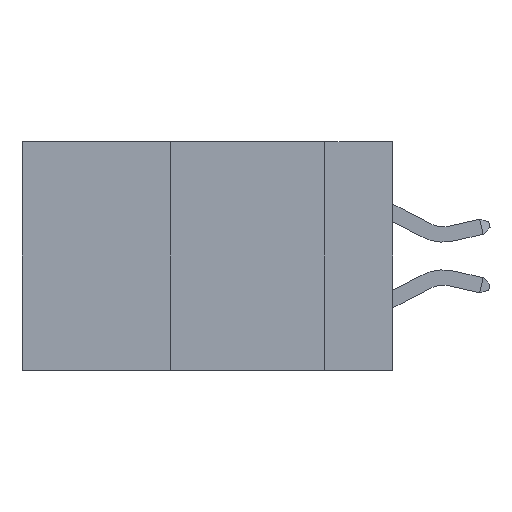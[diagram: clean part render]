
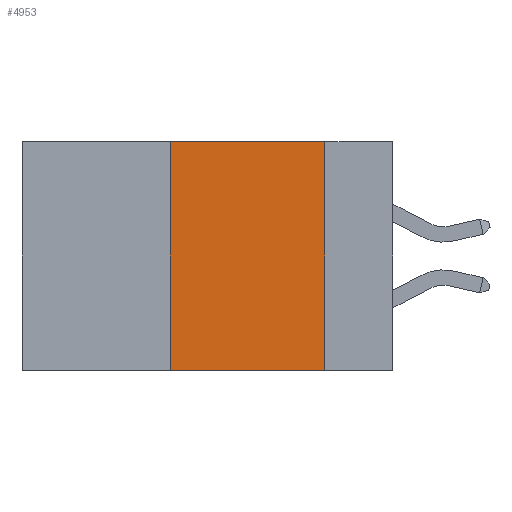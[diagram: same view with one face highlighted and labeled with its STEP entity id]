
A CAD part, left-side view. The second image highlights one B-rep face of the part: STEP entity #4953.
In plain terms, the highlighted planar face has unit normal (-1, 0, 0).
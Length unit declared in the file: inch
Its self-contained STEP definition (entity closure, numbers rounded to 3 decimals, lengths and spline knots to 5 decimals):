
#217 = DIRECTION ( 'NONE',  ( 1., 0., 0. ) ) ;
#533 = CARTESIAN_POINT ( 'NONE',  ( 0., 0.36, -0.37 ) ) ;
#1213 = VERTEX_POINT ( 'NONE', #14336 ) ;
#1267 = DIRECTION ( 'NONE',  ( 0., 0., -1. ) ) ;
#1674 = VECTOR ( 'NONE', #2005, 39.37008 ) ;
#1988 = ORIENTED_EDGE ( 'NONE', *, *, #5839, .F. ) ;
#2005 = DIRECTION ( 'NONE',  ( 0., 0., 1. ) ) ;
#2883 = CARTESIAN_POINT ( 'NONE',  ( 0., 0.36, 0. ) ) ;
#3218 = LINE ( 'NONE', #13666, #1674 ) ;
#3260 = AXIS2_PLACEMENT_3D ( 'NONE', #10325, #217, #1267 ) ;
#3379 = DIRECTION ( 'NONE',  ( 0., -1., 0. ) ) ;
#4046 = EDGE_CURVE ( 'NONE', #10548, #1213, #14669, .T. ) ;
#4181 = EDGE_CURVE ( 'NONE', #4638, #10483, #10303, .T. ) ;
#4638 = VERTEX_POINT ( 'NONE', #533 ) ;
#4953 = ADVANCED_FACE ( 'NONE', ( #10400 ), #5957, .F. ) ;
#5620 = LINE ( 'NONE', #10519, #13855 ) ;
#5839 = EDGE_CURVE ( 'NONE', #1213, #10483, #5620, .T. ) ;
#5957 = PLANE ( 'NONE',  #3260 ) ;
#6471 = DIRECTION ( 'NONE',  ( 0., -1., 0. ) ) ;
#7201 = EDGE_LOOP ( 'NONE', ( #1988, #12500, #8692, #10534 ) ) ;
#8388 = VECTOR ( 'NONE', #3379, 39.37008 ) ;
#8692 = ORIENTED_EDGE ( 'NONE', *, *, #11464, .F. ) ;
#10012 = CARTESIAN_POINT ( 'NONE',  ( 0., 0.6, 0. ) ) ;
#10216 = DIRECTION ( 'NONE',  ( 0., 0., -1. ) ) ;
#10303 = LINE ( 'NONE', #13678, #8388 ) ;
#10325 = CARTESIAN_POINT ( 'NONE',  ( 0., 0.6, 0. ) ) ;
#10400 = FACE_OUTER_BOUND ( 'NONE', #7201, .T. ) ;
#10483 = VERTEX_POINT ( 'NONE', #12084 ) ;
#10519 = CARTESIAN_POINT ( 'NONE',  ( 0., 0.11, 0. ) ) ;
#10534 = ORIENTED_EDGE ( 'NONE', *, *, #4181, .T. ) ;
#10548 = VERTEX_POINT ( 'NONE', #2883 ) ;
#10849 = VECTOR ( 'NONE', #6471, 39.37008 ) ;
#11464 = EDGE_CURVE ( 'NONE', #4638, #10548, #3218, .T. ) ;
#12084 = CARTESIAN_POINT ( 'NONE',  ( 0., 0.11, -0.37 ) ) ;
#12500 = ORIENTED_EDGE ( 'NONE', *, *, #4046, .F. ) ;
#13666 = CARTESIAN_POINT ( 'NONE',  ( 0., 0.36, 0. ) ) ;
#13678 = CARTESIAN_POINT ( 'NONE',  ( 0., 0.6, -0.37 ) ) ;
#13855 = VECTOR ( 'NONE', #10216, 39.37008 ) ;
#14336 = CARTESIAN_POINT ( 'NONE',  ( 0., 0.11, 0. ) ) ;
#14669 = LINE ( 'NONE', #10012, #10849 ) ;
